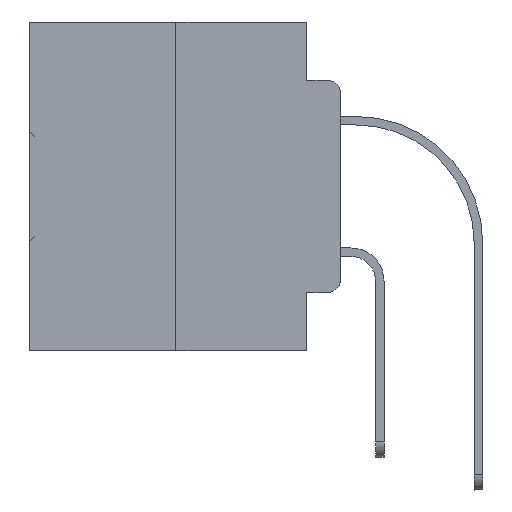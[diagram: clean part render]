
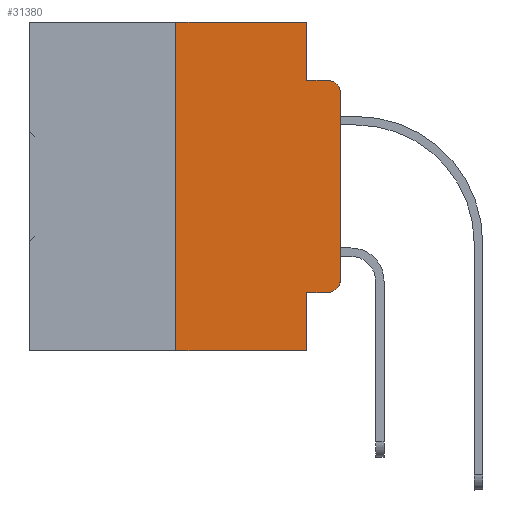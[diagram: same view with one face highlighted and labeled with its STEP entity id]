
A CAD part, left-side view. The second image highlights one B-rep face of the part: STEP entity #31380.
In plain terms, the highlighted planar face has unit normal (-1, 0, 0).
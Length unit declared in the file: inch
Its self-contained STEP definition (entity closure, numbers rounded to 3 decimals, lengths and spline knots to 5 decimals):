
#318 = VECTOR ( 'NONE', #3061, 39.37008 ) ;
#466 = CARTESIAN_POINT ( 'NONE',  ( 0., 0.25, -0.5 ) ) ;
#519 = CARTESIAN_POINT ( 'NONE',  ( 0., 0.051, -0.5 ) ) ;
#906 = LINE ( 'NONE', #21270, #1928 ) ;
#1337 = EDGE_LOOP ( 'NONE', ( #18936, #13008, #14743, #32775, #33029, #32230, #4309, #26409, #13728, #18831 ) ) ;
#1928 = VECTOR ( 'NONE', #32959, 39.37008 ) ;
#2377 = CARTESIAN_POINT ( 'NONE',  ( 0., 0.473, 0. ) ) ;
#2935 = DIRECTION ( 'NONE',  ( 0., 0., -1. ) ) ;
#3052 = VECTOR ( 'NONE', #24424, 39.37008 ) ;
#3061 = DIRECTION ( 'NONE',  ( 0., -1., 0. ) ) ;
#3428 = LINE ( 'NONE', #32304, #318 ) ;
#3962 = CARTESIAN_POINT ( 'NONE',  ( 0., 0.02, -0.1085 ) ) ;
#4040 = CARTESIAN_POINT ( 'NONE',  ( 0., 0.051, -0.0885 ) ) ;
#4309 = ORIENTED_EDGE ( 'NONE', *, *, #22660, .T. ) ;
#5035 = DIRECTION ( 'NONE',  ( 1., 0., 0. ) ) ;
#5358 = CARTESIAN_POINT ( 'NONE',  ( 0., 0., -0.1085 ) ) ;
#5362 = VERTEX_POINT ( 'NONE', #4040 ) ;
#5585 = FACE_OUTER_BOUND ( 'NONE', #1337, .T. ) ;
#5809 = LINE ( 'NONE', #32025, #24757 ) ;
#5929 = EDGE_CURVE ( 'NONE', #33201, #28899, #27303, .T. ) ;
#6215 = DIRECTION ( 'NONE',  ( 0., -1., 0. ) ) ;
#6793 = AXIS2_PLACEMENT_3D ( 'NONE', #3962, #24911, #12639 ) ;
#6868 = CARTESIAN_POINT ( 'NONE',  ( 0., 0.25, 0. ) ) ;
#7354 = EDGE_CURVE ( 'NONE', #5362, #28899, #9151, .T. ) ;
#7595 = EDGE_CURVE ( 'NONE', #7746, #33201, #33489, .T. ) ;
#7731 = AXIS2_PLACEMENT_3D ( 'NONE', #2377, #5035, #2935 ) ;
#7746 = VERTEX_POINT ( 'NONE', #35099 ) ;
#8857 = CARTESIAN_POINT ( 'NONE',  ( 0., 0.473, 0. ) ) ;
#9151 = LINE ( 'NONE', #35376, #9895 ) ;
#9525 = DIRECTION ( 'NONE',  ( 0., -1., 0. ) ) ;
#9895 = VECTOR ( 'NONE', #9525, 39.37008 ) ;
#11628 = EDGE_CURVE ( 'NONE', #27758, #5362, #20959, .T. ) ;
#12639 = DIRECTION ( 'NONE',  ( 0., 0., -1. ) ) ;
#13008 = ORIENTED_EDGE ( 'NONE', *, *, #5929, .T. ) ;
#13007 = EDGE_CURVE ( 'NONE', #19762, #17306, #18364, .T. ) ;
#13728 = ORIENTED_EDGE ( 'NONE', *, *, #37154, .T. ) ;
#14743 = ORIENTED_EDGE ( 'NONE', *, *, #7354, .F. ) ;
#17306 = VERTEX_POINT ( 'NONE', #23324 ) ;
#17755 = CARTESIAN_POINT ( 'NONE',  ( 0., 0.051, 0. ) ) ;
#18364 = LINE ( 'NONE', #6868, #3052 ) ;
#18649 = VECTOR ( 'NONE', #6215, 39.37008 ) ;
#18785 = AXIS2_PLACEMENT_3D ( 'NONE', #21239, #27657, #32745 ) ;
#18831 = ORIENTED_EDGE ( 'NONE', *, *, #27199, .T. ) ;
#18936 = ORIENTED_EDGE ( 'NONE', *, *, #7595, .T. ) ;
#19762 = VERTEX_POINT ( 'NONE', #466 ) ;
#20017 = VECTOR ( 'NONE', #29650, 39.37008 ) ;
#20327 = DIRECTION ( 'NONE',  ( 0., 0., -1. ) ) ;
#20959 = LINE ( 'NONE', #17755, #20017 ) ;
#21239 = CARTESIAN_POINT ( 'NONE',  ( 0., 0.02, -0.3915 ) ) ;
#21270 = CARTESIAN_POINT ( 'NONE',  ( 0., 0.051, -0.4115 ) ) ;
#21557 = CARTESIAN_POINT ( 'NONE',  ( 0., 0.02, -0.4115 ) ) ;
#22660 = EDGE_CURVE ( 'NONE', #19762, #37029, #3428, .T. ) ;
#22899 = CARTESIAN_POINT ( 'NONE',  ( 0., 0.051, -0.4115 ) ) ;
#23005 = VERTEX_POINT ( 'NONE', #22899 ) ;
#23324 = CARTESIAN_POINT ( 'NONE',  ( 0., 0.25, 0. ) ) ;
#23606 = CIRCLE ( 'NONE', #18785, 0.02 ) ;
#24026 = CARTESIAN_POINT ( 'NONE',  ( 0., 0.02, -0.0885 ) ) ;
#24424 = DIRECTION ( 'NONE',  ( 0., 0., 1. ) ) ;
#24757 = VECTOR ( 'NONE', #20327, 39.37008 ) ;
#24911 = DIRECTION ( 'NONE',  ( -1., 0., 0. ) ) ;
#24995 = VECTOR ( 'NONE', #36877, 39.37008 ) ;
#26393 = LINE ( 'NONE', #8857, #18649 ) ;
#26409 = ORIENTED_EDGE ( 'NONE', *, *, #35639, .F. ) ;
#27199 = EDGE_CURVE ( 'NONE', #33469, #7746, #23606, .T. ) ;
#27303 = CIRCLE ( 'NONE', #6793, 0.02 ) ;
#27657 = DIRECTION ( 'NONE',  ( -1., 0., 0. ) ) ;
#27758 = VERTEX_POINT ( 'NONE', #30807 ) ;
#28899 = VERTEX_POINT ( 'NONE', #24026 ) ;
#29604 = EDGE_CURVE ( 'NONE', #17306, #27758, #26393, .T. ) ;
#29650 = DIRECTION ( 'NONE',  ( 0., 0., -1. ) ) ;
#30807 = CARTESIAN_POINT ( 'NONE',  ( 0., 0.051, 0. ) ) ;
#31032 = CARTESIAN_POINT ( 'NONE',  ( 0., 0., 0. ) ) ;
#31077 = PLANE ( 'NONE',  #7731 ) ;
#31380 = ADVANCED_FACE ( 'NONE', ( #5585 ), #31077, .F. ) ;
#32025 = CARTESIAN_POINT ( 'NONE',  ( 0., 0.051, 0. ) ) ;
#32230 = ORIENTED_EDGE ( 'NONE', *, *, #13007, .F. ) ;
#32304 = CARTESIAN_POINT ( 'NONE',  ( 0., 0.473, -0.5 ) ) ;
#32745 = DIRECTION ( 'NONE',  ( 0., 0., -1. ) ) ;
#32775 = ORIENTED_EDGE ( 'NONE', *, *, #11628, .F. ) ;
#32959 = DIRECTION ( 'NONE',  ( 0., -1., 0. ) ) ;
#33029 = ORIENTED_EDGE ( 'NONE', *, *, #29604, .F. ) ;
#33201 = VERTEX_POINT ( 'NONE', #5358 ) ;
#33469 = VERTEX_POINT ( 'NONE', #21557 ) ;
#33489 = LINE ( 'NONE', #31032, #24995 ) ;
#35099 = CARTESIAN_POINT ( 'NONE',  ( 0., 0., -0.3915 ) ) ;
#35376 = CARTESIAN_POINT ( 'NONE',  ( 0., 0.051, -0.0885 ) ) ;
#35639 = EDGE_CURVE ( 'NONE', #23005, #37029, #5809, .T. ) ;
#36877 = DIRECTION ( 'NONE',  ( 0., 0., 1. ) ) ;
#37029 = VERTEX_POINT ( 'NONE', #519 ) ;
#37154 = EDGE_CURVE ( 'NONE', #23005, #33469, #906, .T. ) ;
